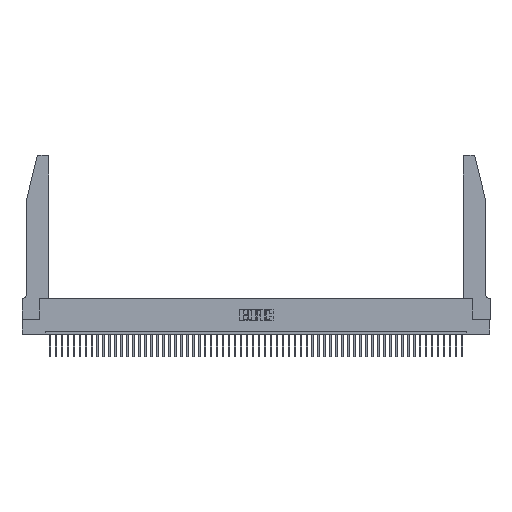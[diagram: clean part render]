
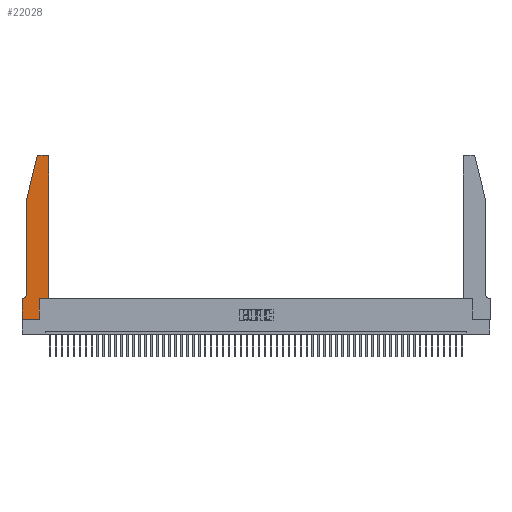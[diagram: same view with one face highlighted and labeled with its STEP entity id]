
A CAD part, top view. The second image highlights one B-rep face of the part: STEP entity #22028.
In plain terms, the highlighted planar face has unit normal (0, 0, 1).
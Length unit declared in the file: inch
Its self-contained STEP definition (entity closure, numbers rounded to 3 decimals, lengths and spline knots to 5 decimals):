
#480 = ORIENTED_EDGE ( 'NONE', *, *, #5664, .T. ) ;
#492 = CARTESIAN_POINT ( 'NONE',  ( 0., 0., 0.37 ) ) ;
#826 = VECTOR ( 'NONE', #12654, 39.37008 ) ;
#856 = CARTESIAN_POINT ( 'NONE',  ( 0.2865, 0.35, 0.37 ) ) ;
#1517 = ORIENTED_EDGE ( 'NONE', *, *, #52877, .T. ) ;
#1747 = CARTESIAN_POINT ( 'NONE',  ( 0.2865, 0.35, 0.37 ) ) ;
#2315 = CIRCLE ( 'NONE', #31422, 0.03 ) ;
#3197 = DIRECTION ( 'NONE',  ( 1., 0., 0. ) ) ;
#3287 = DIRECTION ( 'NONE',  ( 1., 0., 0. ) ) ;
#3913 = EDGE_CURVE ( 'NONE', #38639, #46463, #14608, .T. ) ;
#4144 = DIRECTION ( 'NONE',  ( -1., 0., 0. ) ) ;
#4152 = CARTESIAN_POINT ( 'NONE',  ( 0.0755, 2., 0.37 ) ) ;
#4243 = DIRECTION ( 'NONE',  ( 1., 0., 0. ) ) ;
#5574 = CARTESIAN_POINT ( 'NONE',  ( 0.4505, 2.72, 0.37 ) ) ;
#5653 = EDGE_CURVE ( 'NONE', #17073, #37824, #48806, .T. ) ;
#5664 = EDGE_CURVE ( 'NONE', #6479, #32699, #49449, .T. ) ;
#6479 = VERTEX_POINT ( 'NONE', #6778 ) ;
#6778 = CARTESIAN_POINT ( 'NONE',  ( 0.4205, 2.75, 0.37 ) ) ;
#7400 = VECTOR ( 'NONE', #47989, 39.37008 ) ;
#7844 = VERTEX_POINT ( 'NONE', #52082 ) ;
#8028 = CARTESIAN_POINT ( 'NONE',  ( 0.2865, 0., 0.37 ) ) ;
#8456 = EDGE_CURVE ( 'NONE', #32978, #6479, #35438, .T. ) ;
#9120 = EDGE_CURVE ( 'NONE', #32699, #51534, #2315, .T. ) ;
#9541 = ORIENTED_EDGE ( 'NONE', *, *, #44443, .T. ) ;
#10397 = EDGE_CURVE ( 'NONE', #42321, #17073, #38258, .T. ) ;
#10476 = FACE_OUTER_BOUND ( 'NONE', #35951, .T. ) ;
#10573 = CARTESIAN_POINT ( 'NONE',  ( 0.2605, 2.75, 0.37 ) ) ;
#11914 = CARTESIAN_POINT ( 'NONE',  ( 0.25487, 2.72718, 0.37 ) ) ;
#11997 = EDGE_CURVE ( 'NONE', #32199, #42321, #18710, .T. ) ;
#12085 = AXIS2_PLACEMENT_3D ( 'NONE', #15890, #48422, #52818 ) ;
#12514 = ORIENTED_EDGE ( 'NONE', *, *, #8456, .T. ) ;
#12654 = DIRECTION ( 'NONE',  ( -0.239, -0.971, 0. ) ) ;
#14608 = LINE ( 'NONE', #43606, #41145 ) ;
#14779 = EDGE_CURVE ( 'NONE', #7844, #32199, #43708, .T. ) ;
#14887 = CARTESIAN_POINT ( 'NONE',  ( 0., 0.35, 0.37 ) ) ;
#15450 = DIRECTION ( 'NONE',  ( 1., 0., 0. ) ) ;
#15890 = CARTESIAN_POINT ( 'NONE',  ( 0.4205, 2.72, 0.37 ) ) ;
#15913 = DIRECTION ( 'NONE',  ( -1., 0., 0. ) ) ;
#16258 = CARTESIAN_POINT ( 'NONE',  ( 0.0755, 0.35, 0.37 ) ) ;
#16662 = ORIENTED_EDGE ( 'NONE', *, *, #3913, .T. ) ;
#17073 = VERTEX_POINT ( 'NONE', #8028 ) ;
#18231 = PLANE ( 'NONE',  #49219 ) ;
#18710 = LINE ( 'NONE', #52221, #42618 ) ;
#19081 = DIRECTION ( 'NONE',  ( -1., 0., 0. ) ) ;
#19194 = ORIENTED_EDGE ( 'NONE', *, *, #11997, .T. ) ;
#19240 = DIRECTION ( 'NONE',  ( 0., -1., 0. ) ) ;
#19863 = VECTOR ( 'NONE', #15913, 39.37008 ) ;
#20564 = CARTESIAN_POINT ( 'NONE',  ( 0.284, 2.75, 0.37 ) ) ;
#20646 = CARTESIAN_POINT ( 'NONE',  ( 0.0055, 0.42, 0.37 ) ) ;
#22028 = ADVANCED_FACE ( 'NONE', ( #10476 ), #18231, .T. ) ;
#23324 = DIRECTION ( 'NONE',  ( 0., 0., 1. ) ) ;
#23882 = CARTESIAN_POINT ( 'NONE',  ( 0., 0.35, 0.37 ) ) ;
#25264 = VECTOR ( 'NONE', #40182, 39.37008 ) ;
#25418 = VECTOR ( 'NONE', #15450, 39.37008 ) ;
#27193 = CARTESIAN_POINT ( 'NONE',  ( 0., 0., 0.37 ) ) ;
#27440 = VECTOR ( 'NONE', #19081, 39.37008 ) ;
#27569 = EDGE_CURVE ( 'NONE', #37824, #51671, #45540, .T. ) ;
#28140 = VECTOR ( 'NONE', #4243, 39.37008 ) ;
#29066 = EDGE_CURVE ( 'NONE', #46463, #7844, #37289, .T. ) ;
#29801 = CARTESIAN_POINT ( 'NONE',  ( 0.0755, 0.42, 0.37 ) ) ;
#31057 = LINE ( 'NONE', #35803, #25264 ) ;
#31136 = ORIENTED_EDGE ( 'NONE', *, *, #29066, .T. ) ;
#31422 = AXIS2_PLACEMENT_3D ( 'NONE', #49490, #44539, #3287 ) ;
#32199 = VERTEX_POINT ( 'NONE', #14887 ) ;
#32699 = VERTEX_POINT ( 'NONE', #20564 ) ;
#32978 = VERTEX_POINT ( 'NONE', #5574 ) ;
#35438 = CIRCLE ( 'NONE', #12085, 0.03 ) ;
#35803 = CARTESIAN_POINT ( 'NONE',  ( 0.4505, 0.35, 0.37 ) ) ;
#35951 = EDGE_LOOP ( 'NONE', ( #480, #37946, #1517, #16662, #31136, #36652, #19194, #52561, #48026, #43199, #9541, #12514 ) ) ;
#36652 = ORIENTED_EDGE ( 'NONE', *, *, #14779, .T. ) ;
#37289 = CIRCLE ( 'NONE', #53422, 0.07 ) ;
#37309 = CARTESIAN_POINT ( 'NONE',  ( 0.4505, 0.35, 0.37 ) ) ;
#37824 = VERTEX_POINT ( 'NONE', #856 ) ;
#37946 = ORIENTED_EDGE ( 'NONE', *, *, #9120, .T. ) ;
#38258 = LINE ( 'NONE', #27193, #25418 ) ;
#38639 = VERTEX_POINT ( 'NONE', #4152 ) ;
#40182 = DIRECTION ( 'NONE',  ( 0., 1., 0. ) ) ;
#40557 = LINE ( 'NONE', #41048, #826 ) ;
#41048 = CARTESIAN_POINT ( 'NONE',  ( 0.0755, 2., 0.37 ) ) ;
#41145 = VECTOR ( 'NONE', #19240, 39.37008 ) ;
#42321 = VERTEX_POINT ( 'NONE', #492 ) ;
#42618 = VECTOR ( 'NONE', #48224, 39.37008 ) ;
#43199 = ORIENTED_EDGE ( 'NONE', *, *, #27569, .T. ) ;
#43606 = CARTESIAN_POINT ( 'NONE',  ( 0.0755, 2., 0.37 ) ) ;
#43708 = LINE ( 'NONE', #16258, #19863 ) ;
#44443 = EDGE_CURVE ( 'NONE', #51671, #32978, #31057, .T. ) ;
#44539 = DIRECTION ( 'NONE',  ( 0., 0., 1. ) ) ;
#45491 = CARTESIAN_POINT ( 'NONE',  ( 0.4505, 0.35, 0.37 ) ) ;
#45540 = LINE ( 'NONE', #45491, #28140 ) ;
#46463 = VERTEX_POINT ( 'NONE', #29801 ) ;
#47989 = DIRECTION ( 'NONE',  ( 0., 1., 0. ) ) ;
#48026 = ORIENTED_EDGE ( 'NONE', *, *, #5653, .T. ) ;
#48224 = DIRECTION ( 'NONE',  ( 0., -1., 0. ) ) ;
#48422 = DIRECTION ( 'NONE',  ( 0., 0., 1. ) ) ;
#48806 = LINE ( 'NONE', #1747, #7400 ) ;
#49219 = AXIS2_PLACEMENT_3D ( 'NONE', #23882, #23324, #3197 ) ;
#49449 = LINE ( 'NONE', #10573, #27440 ) ;
#49490 = CARTESIAN_POINT ( 'NONE',  ( 0.284, 2.72, 0.37 ) ) ;
#49587 = DIRECTION ( 'NONE',  ( 0., 0., -1. ) ) ;
#51534 = VERTEX_POINT ( 'NONE', #11914 ) ;
#51671 = VERTEX_POINT ( 'NONE', #37309 ) ;
#52082 = CARTESIAN_POINT ( 'NONE',  ( 0.0055, 0.35, 0.37 ) ) ;
#52221 = CARTESIAN_POINT ( 'NONE',  ( 0., 0., 0.37 ) ) ;
#52561 = ORIENTED_EDGE ( 'NONE', *, *, #10397, .T. ) ;
#52818 = DIRECTION ( 'NONE',  ( 1., 0., 0. ) ) ;
#52877 = EDGE_CURVE ( 'NONE', #51534, #38639, #40557, .T. ) ;
#53422 = AXIS2_PLACEMENT_3D ( 'NONE', #20646, #49587, #4144 ) ;
